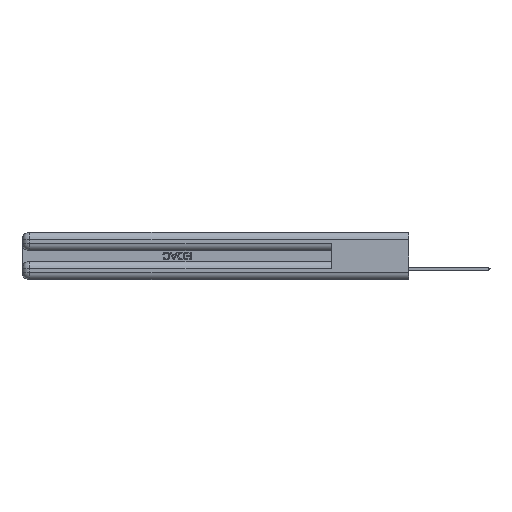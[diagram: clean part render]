
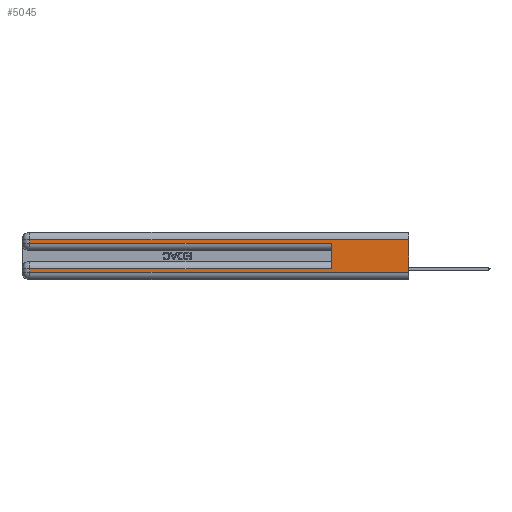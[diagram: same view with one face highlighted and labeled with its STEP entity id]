
A CAD part, left-side view. The second image highlights one B-rep face of the part: STEP entity #5045.
In plain terms, the highlighted planar face has unit normal (-1, 0, 0).
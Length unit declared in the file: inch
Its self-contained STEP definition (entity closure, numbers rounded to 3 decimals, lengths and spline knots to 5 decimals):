
#3177 = LINE ( 'NONE', #40824, #15658 ) ;
#3192 = VERTEX_POINT ( 'NONE', #18856 ) ;
#3544 = CARTESIAN_POINT ( 'NONE',  ( 0., 2.94, 0.285 ) ) ;
#4250 = CARTESIAN_POINT ( 'NONE',  ( 0., 2.94, 0.37 ) ) ;
#4865 = CARTESIAN_POINT ( 'NONE',  ( 0., 0.6, 0.145 ) ) ;
#5045 = ADVANCED_FACE ( 'NONE', ( #39798 ), #13655, .F. ) ;
#5516 = LINE ( 'NONE', #34232, #22950 ) ;
#6190 = DIRECTION ( 'NONE',  ( 1., 0., 0. ) ) ;
#6198 = VERTEX_POINT ( 'NONE', #36656 ) ;
#6712 = CARTESIAN_POINT ( 'NONE',  ( 0., 2.94, 0.37 ) ) ;
#8578 = EDGE_CURVE ( 'NONE', #3192, #32463, #3177, .T. ) ;
#8848 = DIRECTION ( 'NONE',  ( 0., 0., 1. ) ) ;
#9711 = DIRECTION ( 'NONE',  ( 0., 0., -1. ) ) ;
#10633 = EDGE_CURVE ( 'NONE', #6198, #18688, #19396, .T. ) ;
#12011 = VECTOR ( 'NONE', #41139, 39.37008 ) ;
#12404 = DIRECTION ( 'NONE',  ( 0., -1., 0. ) ) ;
#12663 = ORIENTED_EDGE ( 'NONE', *, *, #8578, .F. ) ;
#13103 = LINE ( 'NONE', #6712, #39543 ) ;
#13384 = ORIENTED_EDGE ( 'NONE', *, *, #38548, .T. ) ;
#13655 = PLANE ( 'NONE',  #44785 ) ;
#13871 = LINE ( 'NONE', #38804, #30742 ) ;
#14604 = CARTESIAN_POINT ( 'NONE',  ( 0., 2.94, 0.085 ) ) ;
#14797 = DIRECTION ( 'NONE',  ( 0., 1., 0. ) ) ;
#15005 = ORIENTED_EDGE ( 'NONE', *, *, #36374, .T. ) ;
#15658 = VECTOR ( 'NONE', #37690, 39.37008 ) ;
#16373 = LINE ( 'NONE', #4250, #16922 ) ;
#16922 = VECTOR ( 'NONE', #32311, 39.37008 ) ;
#17038 = CARTESIAN_POINT ( 'NONE',  ( 0., 0., 0.31 ) ) ;
#17481 = DIRECTION ( 'NONE',  ( 0., -1., 0. ) ) ;
#18648 = EDGE_CURVE ( 'NONE', #43332, #18688, #5516, .T. ) ;
#18688 = VERTEX_POINT ( 'NONE', #39740 ) ;
#18842 = VECTOR ( 'NONE', #8848, 39.37008 ) ;
#18856 = CARTESIAN_POINT ( 'NONE',  ( 0., 0., 0.31 ) ) ;
#19046 = LINE ( 'NONE', #22291, #35687 ) ;
#19396 = LINE ( 'NONE', #4865, #18842 ) ;
#19773 = EDGE_CURVE ( 'NONE', #32322, #43332, #16373, .T. ) ;
#19808 = CARTESIAN_POINT ( 'NONE',  ( 0., 0., 0.06 ) ) ;
#20676 = EDGE_CURVE ( 'NONE', #28334, #32463, #19046, .T. ) ;
#22291 = CARTESIAN_POINT ( 'NONE',  ( 0., 0., 0.06 ) ) ;
#22950 = VECTOR ( 'NONE', #17481, 39.37008 ) ;
#28334 = VERTEX_POINT ( 'NONE', #39907 ) ;
#28487 = VERTEX_POINT ( 'NONE', #14604 ) ;
#30582 = ORIENTED_EDGE ( 'NONE', *, *, #41698, .T. ) ;
#30742 = VECTOR ( 'NONE', #14797, 39.37008 ) ;
#30984 = CARTESIAN_POINT ( 'NONE',  ( 0., 2.94, 0.31 ) ) ;
#31443 = ORIENTED_EDGE ( 'NONE', *, *, #20676, .T. ) ;
#32003 = LINE ( 'NONE', #17038, #12011 ) ;
#32311 = DIRECTION ( 'NONE',  ( 0., 0., -1. ) ) ;
#32322 = VERTEX_POINT ( 'NONE', #30984 ) ;
#32463 = VERTEX_POINT ( 'NONE', #19808 ) ;
#34232 = CARTESIAN_POINT ( 'NONE',  ( 0., 0., 0.285 ) ) ;
#34388 = DIRECTION ( 'NONE',  ( 0., 0., -1. ) ) ;
#35427 = EDGE_LOOP ( 'NONE', ( #12663, #13384, #40930, #41460, #43696, #30582, #15005, #31443 ) ) ;
#35687 = VECTOR ( 'NONE', #12404, 39.37008 ) ;
#36374 = EDGE_CURVE ( 'NONE', #28487, #28334, #13103, .T. ) ;
#36656 = CARTESIAN_POINT ( 'NONE',  ( 0., 0.6, 0.085 ) ) ;
#37376 = CARTESIAN_POINT ( 'NONE',  ( 0., 0., 0.37 ) ) ;
#37690 = DIRECTION ( 'NONE',  ( 0., 0., -1. ) ) ;
#38548 = EDGE_CURVE ( 'NONE', #3192, #32322, #32003, .T. ) ;
#38804 = CARTESIAN_POINT ( 'NONE',  ( 0., 0., 0.085 ) ) ;
#39543 = VECTOR ( 'NONE', #34388, 39.37008 ) ;
#39740 = CARTESIAN_POINT ( 'NONE',  ( 0., 0.6, 0.285 ) ) ;
#39798 = FACE_OUTER_BOUND ( 'NONE', #35427, .T. ) ;
#39907 = CARTESIAN_POINT ( 'NONE',  ( 0., 2.94, 0.06 ) ) ;
#40824 = CARTESIAN_POINT ( 'NONE',  ( 0., 0., 0.37 ) ) ;
#40930 = ORIENTED_EDGE ( 'NONE', *, *, #19773, .T. ) ;
#41139 = DIRECTION ( 'NONE',  ( 0., 1., 0. ) ) ;
#41460 = ORIENTED_EDGE ( 'NONE', *, *, #18648, .T. ) ;
#41698 = EDGE_CURVE ( 'NONE', #6198, #28487, #13871, .T. ) ;
#43332 = VERTEX_POINT ( 'NONE', #3544 ) ;
#43696 = ORIENTED_EDGE ( 'NONE', *, *, #10633, .F. ) ;
#44785 = AXIS2_PLACEMENT_3D ( 'NONE', #37376, #6190, #9711 ) ;
